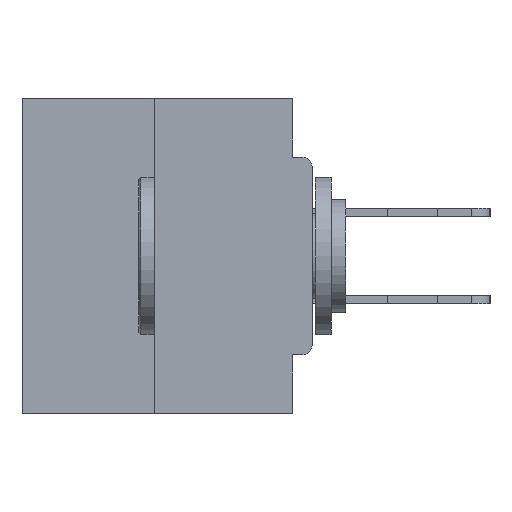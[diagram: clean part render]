
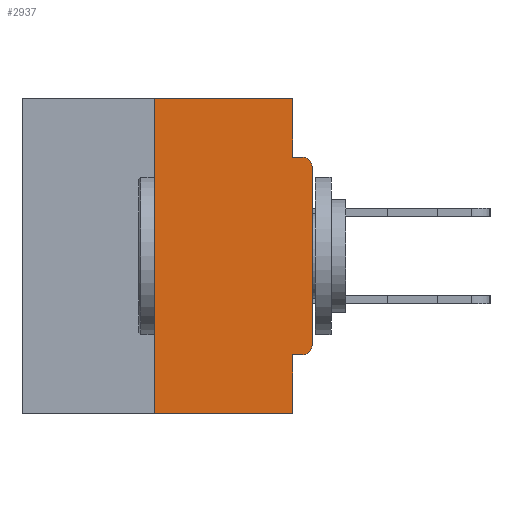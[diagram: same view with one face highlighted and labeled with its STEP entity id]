
A CAD part, left-side view. The second image highlights one B-rep face of the part: STEP entity #2937.
In plain terms, the highlighted planar face has unit normal (-1, 0, 0).
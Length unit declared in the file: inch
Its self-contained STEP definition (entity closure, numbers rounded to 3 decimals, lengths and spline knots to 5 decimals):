
#142 = VERTEX_POINT ( 'NONE', #20337 ) ;
#387 = EDGE_CURVE ( 'NONE', #142, #21671, #33884, .T. ) ;
#948 = DIRECTION ( 'NONE',  ( 0., 1., 0. ) ) ;
#1562 = DIRECTION ( 'NONE',  ( 0., -1., 0. ) ) ;
#1822 = CARTESIAN_POINT ( 'NONE',  ( 0., 0., 0. ) ) ;
#1881 = VERTEX_POINT ( 'NONE', #32266 ) ;
#1935 = CARTESIAN_POINT ( 'NONE',  ( 0., 0.031, -0.4065 ) ) ;
#2155 = AXIS2_PLACEMENT_3D ( 'NONE', #22692, #14433, #14089 ) ;
#2450 = CARTESIAN_POINT ( 'NONE',  ( 0., 0.031, -0.0935 ) ) ;
#2937 = ADVANCED_FACE ( 'NONE', ( #10935 ), #23179, .F. ) ;
#3022 = CIRCLE ( 'NONE', #32342, 0.015 ) ;
#3537 = DIRECTION ( 'NONE',  ( 0., -1., 0. ) ) ;
#3862 = VECTOR ( 'NONE', #35649, 39.37008 ) ;
#3968 = DIRECTION ( 'NONE',  ( -1., 0., 0. ) ) ;
#4017 = EDGE_CURVE ( 'NONE', #142, #9820, #28251, .T. ) ;
#4731 = CARTESIAN_POINT ( 'NONE',  ( 0., 0.031, 0. ) ) ;
#4772 = LINE ( 'NONE', #1822, #3862 ) ;
#5306 = LINE ( 'NONE', #32638, #9718 ) ;
#6962 = VECTOR ( 'NONE', #23906, 39.37008 ) ;
#7001 = LINE ( 'NONE', #30212, #28403 ) ;
#7274 = ORIENTED_EDGE ( 'NONE', *, *, #16684, .F. ) ;
#7406 = EDGE_CURVE ( 'NONE', #27963, #28785, #19220, .T. ) ;
#8286 = LINE ( 'NONE', #32289, #6962 ) ;
#9047 = CARTESIAN_POINT ( 'NONE',  ( 0., 0., -0.1085 ) ) ;
#9123 = CARTESIAN_POINT ( 'NONE',  ( 0., 0.46, -0.5 ) ) ;
#9688 = LINE ( 'NONE', #9123, #16397 ) ;
#9718 = VECTOR ( 'NONE', #29523, 39.37008 ) ;
#9820 = VERTEX_POINT ( 'NONE', #1935 ) ;
#10935 = FACE_OUTER_BOUND ( 'NONE', #33908, .T. ) ;
#11044 = EDGE_CURVE ( 'NONE', #28785, #36016, #22925, .T. ) ;
#12073 = CARTESIAN_POINT ( 'NONE',  ( 0., 0., -0.4065 ) ) ;
#12269 = VECTOR ( 'NONE', #19648, 39.37008 ) ;
#13563 = DIRECTION ( 'NONE',  ( 0., 0., -1. ) ) ;
#13772 = ORIENTED_EDGE ( 'NONE', *, *, #17736, .T. ) ;
#14089 = DIRECTION ( 'NONE',  ( 0., 0., -1. ) ) ;
#14433 = DIRECTION ( 'NONE',  ( 1., 0., 0. ) ) ;
#15718 = VERTEX_POINT ( 'NONE', #9047 ) ;
#15834 = DIRECTION ( 'NONE',  ( -1., 0., 0. ) ) ;
#16397 = VECTOR ( 'NONE', #3537, 39.37008 ) ;
#16684 = EDGE_CURVE ( 'NONE', #9820, #17033, #5306, .T. ) ;
#17033 = VERTEX_POINT ( 'NONE', #28639 ) ;
#17129 = ORIENTED_EDGE ( 'NONE', *, *, #4017, .F. ) ;
#17736 = EDGE_CURVE ( 'NONE', #19106, #17033, #9688, .T. ) ;
#18295 = VECTOR ( 'NONE', #33826, 39.37008 ) ;
#18544 = EDGE_CURVE ( 'NONE', #15718, #36016, #3022, .T. ) ;
#18963 = EDGE_CURVE ( 'NONE', #21671, #15718, #4772, .T. ) ;
#19020 = EDGE_CURVE ( 'NONE', #1881, #27963, #7001, .T. ) ;
#19106 = VERTEX_POINT ( 'NONE', #19848 ) ;
#19220 = LINE ( 'NONE', #24795, #18295 ) ;
#19290 = EDGE_CURVE ( 'NONE', #19106, #1881, #8286, .T. ) ;
#19648 = DIRECTION ( 'NONE',  ( 0., -1., 0. ) ) ;
#19848 = CARTESIAN_POINT ( 'NONE',  ( 0., 0.25, -0.5 ) ) ;
#20337 = CARTESIAN_POINT ( 'NONE',  ( 0., 0.015, -0.4065 ) ) ;
#20897 = AXIS2_PLACEMENT_3D ( 'NONE', #21302, #15834, #13563 ) ;
#21302 = CARTESIAN_POINT ( 'NONE',  ( 0., 0.015, -0.3915 ) ) ;
#21671 = VERTEX_POINT ( 'NONE', #35170 ) ;
#22692 = CARTESIAN_POINT ( 'NONE',  ( 0., 0.46, 0. ) ) ;
#22925 = LINE ( 'NONE', #25226, #12269 ) ;
#23179 = PLANE ( 'NONE',  #2155 ) ;
#23906 = DIRECTION ( 'NONE',  ( 0., 0., 1. ) ) ;
#24775 = ORIENTED_EDGE ( 'NONE', *, *, #19290, .F. ) ;
#24795 = CARTESIAN_POINT ( 'NONE',  ( 0., 0.031, 0. ) ) ;
#25226 = CARTESIAN_POINT ( 'NONE',  ( 0., 0., -0.0935 ) ) ;
#26509 = CARTESIAN_POINT ( 'NONE',  ( 0., 0.015, -0.0935 ) ) ;
#26856 = ORIENTED_EDGE ( 'NONE', *, *, #18544, .T. ) ;
#27010 = DIRECTION ( 'NONE',  ( 0., 0., -1. ) ) ;
#27264 = CARTESIAN_POINT ( 'NONE',  ( 0., 0.015, -0.1085 ) ) ;
#27307 = ORIENTED_EDGE ( 'NONE', *, *, #7406, .F. ) ;
#27963 = VERTEX_POINT ( 'NONE', #4731 ) ;
#28122 = ORIENTED_EDGE ( 'NONE', *, *, #19020, .F. ) ;
#28251 = LINE ( 'NONE', #12073, #32715 ) ;
#28403 = VECTOR ( 'NONE', #1562, 39.37008 ) ;
#28639 = CARTESIAN_POINT ( 'NONE',  ( 0., 0.031, -0.5 ) ) ;
#28785 = VERTEX_POINT ( 'NONE', #2450 ) ;
#29258 = ORIENTED_EDGE ( 'NONE', *, *, #387, .T. ) ;
#29523 = DIRECTION ( 'NONE',  ( 0., 0., -1. ) ) ;
#30107 = ORIENTED_EDGE ( 'NONE', *, *, #11044, .F. ) ;
#30212 = CARTESIAN_POINT ( 'NONE',  ( 0., 0.46, 0. ) ) ;
#32266 = CARTESIAN_POINT ( 'NONE',  ( 0., 0.25, 0. ) ) ;
#32289 = CARTESIAN_POINT ( 'NONE',  ( 0., 0.25, 0. ) ) ;
#32342 = AXIS2_PLACEMENT_3D ( 'NONE', #27264, #3968, #27010 ) ;
#32638 = CARTESIAN_POINT ( 'NONE',  ( 0., 0.031, -0.5 ) ) ;
#32715 = VECTOR ( 'NONE', #948, 39.37008 ) ;
#33826 = DIRECTION ( 'NONE',  ( 0., 0., -1. ) ) ;
#33884 = CIRCLE ( 'NONE', #20897, 0.015 ) ;
#33908 = EDGE_LOOP ( 'NONE', ( #28122, #24775, #13772, #7274, #17129, #29258, #35240, #26856, #30107, #27307 ) ) ;
#35170 = CARTESIAN_POINT ( 'NONE',  ( 0., 0., -0.3915 ) ) ;
#35240 = ORIENTED_EDGE ( 'NONE', *, *, #18963, .T. ) ;
#35649 = DIRECTION ( 'NONE',  ( 0., 0., 1. ) ) ;
#36016 = VERTEX_POINT ( 'NONE', #26509 ) ;
